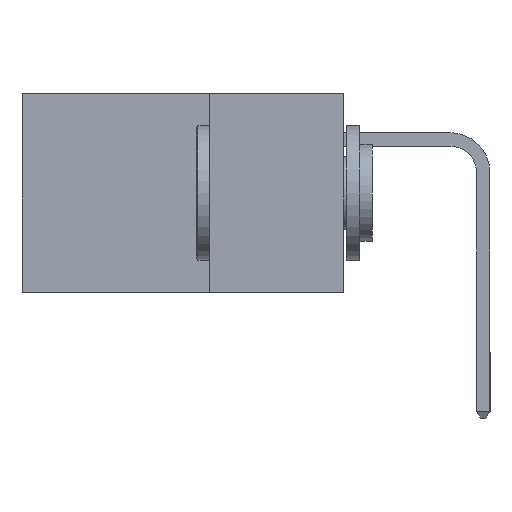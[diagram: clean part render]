
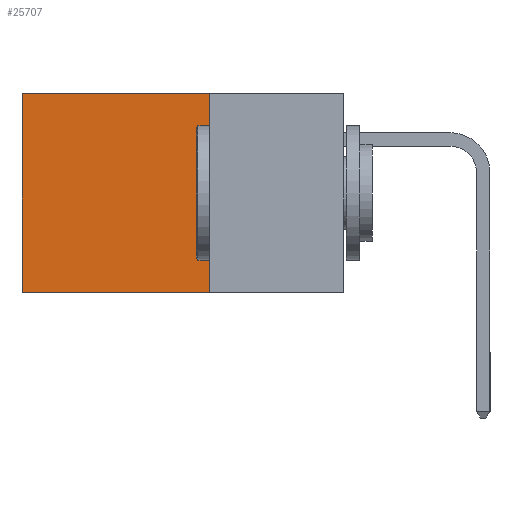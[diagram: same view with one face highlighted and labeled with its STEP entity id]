
A CAD part, left-side view. The second image highlights one B-rep face of the part: STEP entity #25707.
In plain terms, the highlighted planar face has unit normal (-1, 0, 0).
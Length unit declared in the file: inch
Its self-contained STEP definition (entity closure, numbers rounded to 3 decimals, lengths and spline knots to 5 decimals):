
#129 = LINE ( 'NONE', #18366, #14586 ) ;
#207 = AXIS2_PLACEMENT_3D ( 'NONE', #2402, #21359, #4355 ) ;
#1736 = CARTESIAN_POINT ( 'NONE',  ( 0.298, 0.25, 0. ) ) ;
#2402 = CARTESIAN_POINT ( 'NONE',  ( 0.298, 0.25, 0. ) ) ;
#3242 = LINE ( 'NONE', #21377, #28470 ) ;
#3541 = CARTESIAN_POINT ( 'NONE',  ( 0.298, 0.25, -0.37 ) ) ;
#3654 = EDGE_CURVE ( 'NONE', #13787, #5266, #3242, .T. ) ;
#3907 = DIRECTION ( 'NONE',  ( 0., 1., 0. ) ) ;
#4355 = DIRECTION ( 'NONE',  ( 0., 0., -1. ) ) ;
#4766 = PLANE ( 'NONE',  #207 ) ;
#5266 = VERTEX_POINT ( 'NONE', #3541 ) ;
#7574 = ORIENTED_EDGE ( 'NONE', *, *, #26456, .T. ) ;
#8314 = FACE_OUTER_BOUND ( 'NONE', #13176, .T. ) ;
#8902 = DIRECTION ( 'NONE',  ( 0., 0., -1. ) ) ;
#9636 = VERTEX_POINT ( 'NONE', #11884 ) ;
#11884 = CARTESIAN_POINT ( 'NONE',  ( 0.298, 0.6, 0. ) ) ;
#12467 = CARTESIAN_POINT ( 'NONE',  ( 0.298, 0.25, -0.37 ) ) ;
#12928 = CARTESIAN_POINT ( 'NONE',  ( 0.298, 0.6, -0.37 ) ) ;
#13176 = EDGE_LOOP ( 'NONE', ( #7574, #27944, #13980, #16620 ) ) ;
#13787 = VERTEX_POINT ( 'NONE', #28158 ) ;
#13980 = ORIENTED_EDGE ( 'NONE', *, *, #3654, .F. ) ;
#14093 = LINE ( 'NONE', #12467, #25884 ) ;
#14586 = VECTOR ( 'NONE', #8902, 39.37008 ) ;
#16620 = ORIENTED_EDGE ( 'NONE', *, *, #30282, .T. ) ;
#18366 = CARTESIAN_POINT ( 'NONE',  ( 0.298, 0.6, 0. ) ) ;
#19741 = DIRECTION ( 'NONE',  ( 0., 1., 0. ) ) ;
#19790 = VERTEX_POINT ( 'NONE', #12928 ) ;
#21359 = DIRECTION ( 'NONE',  ( 1., 0., 0. ) ) ;
#21377 = CARTESIAN_POINT ( 'NONE',  ( 0.298, 0.25, 0. ) ) ;
#21935 = VECTOR ( 'NONE', #3907, 39.37008 ) ;
#23040 = EDGE_CURVE ( 'NONE', #5266, #19790, #14093, .T. ) ;
#23714 = DIRECTION ( 'NONE',  ( 0., 0., -1. ) ) ;
#25210 = LINE ( 'NONE', #1736, #21935 ) ;
#25707 = ADVANCED_FACE ( 'NONE', ( #8314 ), #4766, .F. ) ;
#25884 = VECTOR ( 'NONE', #19741, 39.37008 ) ;
#26456 = EDGE_CURVE ( 'NONE', #9636, #19790, #129, .T. ) ;
#27944 = ORIENTED_EDGE ( 'NONE', *, *, #23040, .F. ) ;
#28158 = CARTESIAN_POINT ( 'NONE',  ( 0.298, 0.25, 0. ) ) ;
#28470 = VECTOR ( 'NONE', #23714, 39.37008 ) ;
#30282 = EDGE_CURVE ( 'NONE', #13787, #9636, #25210, .T. ) ;
